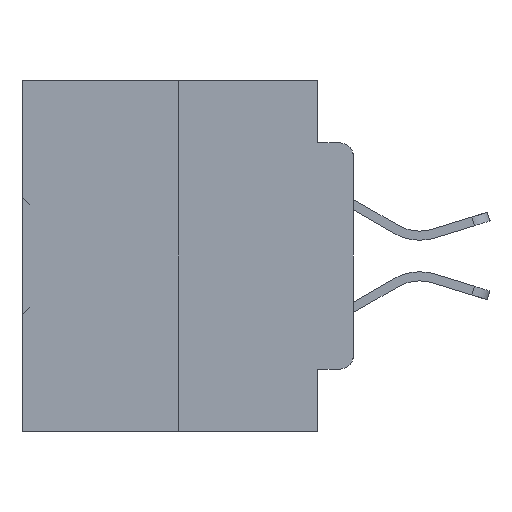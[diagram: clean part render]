
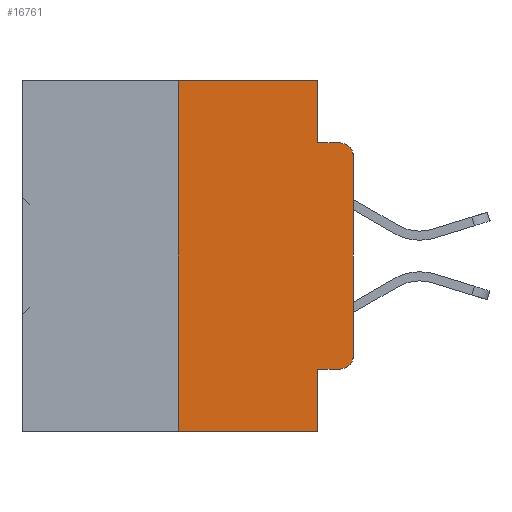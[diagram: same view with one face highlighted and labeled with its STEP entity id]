
A CAD part, left-side view. The second image highlights one B-rep face of the part: STEP entity #16761.
In plain terms, the highlighted planar face has unit normal (-1, 0, 0).
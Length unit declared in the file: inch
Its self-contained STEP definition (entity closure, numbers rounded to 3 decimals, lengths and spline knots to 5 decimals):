
#133 = CIRCLE ( 'NONE', #14691, 0.02 ) ;
#994 = CARTESIAN_POINT ( 'NONE',  ( 0., 0., -0.1085 ) ) ;
#1958 = DIRECTION ( 'NONE',  ( 0., 0., -1. ) ) ;
#3213 = AXIS2_PLACEMENT_3D ( 'NONE', #35539, #20126, #1958 ) ;
#3686 = DIRECTION ( 'NONE',  ( 0., -1., 0. ) ) ;
#3737 = ORIENTED_EDGE ( 'NONE', *, *, #10843, .F. ) ;
#4985 = ORIENTED_EDGE ( 'NONE', *, *, #38586, .T. ) ;
#5687 = EDGE_CURVE ( 'NONE', #9341, #24682, #8997, .T. ) ;
#6096 = VECTOR ( 'NONE', #7437, 39.37008 ) ;
#6361 = VERTEX_POINT ( 'NONE', #33313 ) ;
#6508 = VERTEX_POINT ( 'NONE', #19137 ) ;
#6543 = DIRECTION ( 'NONE',  ( 0., 0., -1. ) ) ;
#7009 = VECTOR ( 'NONE', #31054, 39.37008 ) ;
#7123 = ORIENTED_EDGE ( 'NONE', *, *, #9304, .F. ) ;
#7395 = DIRECTION ( 'NONE',  ( 0., 0., 1. ) ) ;
#7437 = DIRECTION ( 'NONE',  ( 0., 0., -1. ) ) ;
#7978 = FACE_OUTER_BOUND ( 'NONE', #35355, .T. ) ;
#8255 = CARTESIAN_POINT ( 'NONE',  ( 0., 0.051, -0.0885 ) ) ;
#8697 = CIRCLE ( 'NONE', #19473, 0.02 ) ;
#8997 = LINE ( 'NONE', #34598, #26923 ) ;
#9304 = EDGE_CURVE ( 'NONE', #36418, #6508, #15441, .T. ) ;
#9341 = VERTEX_POINT ( 'NONE', #22142 ) ;
#9739 = DIRECTION ( 'NONE',  ( -1., 0., 0. ) ) ;
#10552 = VECTOR ( 'NONE', #22380, 39.37008 ) ;
#10807 = EDGE_CURVE ( 'NONE', #20731, #6508, #11178, .T. ) ;
#10843 = EDGE_CURVE ( 'NONE', #20731, #35156, #24313, .T. ) ;
#11178 = LINE ( 'NONE', #24862, #33299 ) ;
#12107 = EDGE_CURVE ( 'NONE', #24682, #6361, #133, .T. ) ;
#12448 = DIRECTION ( 'NONE',  ( 0., 0., -1. ) ) ;
#13386 = CARTESIAN_POINT ( 'NONE',  ( 0., 0.02, -0.1085 ) ) ;
#13577 = CARTESIAN_POINT ( 'NONE',  ( 0., 0.051, 0. ) ) ;
#14691 = AXIS2_PLACEMENT_3D ( 'NONE', #13386, #18369, #12448 ) ;
#15061 = CARTESIAN_POINT ( 'NONE',  ( 0., 0.25, 0. ) ) ;
#15441 = LINE ( 'NONE', #29222, #6096 ) ;
#16761 = ADVANCED_FACE ( 'NONE', ( #7978 ), #19984, .F. ) ;
#17739 = CARTESIAN_POINT ( 'NONE',  ( 0., 0.02, -0.4115 ) ) ;
#18055 = ORIENTED_EDGE ( 'NONE', *, *, #31976, .F. ) ;
#18369 = DIRECTION ( 'NONE',  ( -1., 0., 0. ) ) ;
#18503 = CARTESIAN_POINT ( 'NONE',  ( 0., 0.473, 0. ) ) ;
#19137 = CARTESIAN_POINT ( 'NONE',  ( 0., 0.051, -0.5 ) ) ;
#19473 = AXIS2_PLACEMENT_3D ( 'NONE', #27525, #9739, #36559 ) ;
#19984 = PLANE ( 'NONE',  #3213 ) ;
#20126 = DIRECTION ( 'NONE',  ( 1., 0., 0. ) ) ;
#20128 = VECTOR ( 'NONE', #6543, 39.37008 ) ;
#20731 = VERTEX_POINT ( 'NONE', #25980 ) ;
#22142 = CARTESIAN_POINT ( 'NONE',  ( 0., 0., -0.3915 ) ) ;
#22200 = VECTOR ( 'NONE', #29335, 39.37008 ) ;
#22233 = CARTESIAN_POINT ( 'NONE',  ( 0., 0.051, -0.4115 ) ) ;
#22380 = DIRECTION ( 'NONE',  ( 0., -1., 0. ) ) ;
#22462 = ORIENTED_EDGE ( 'NONE', *, *, #12107, .T. ) ;
#22545 = CARTESIAN_POINT ( 'NONE',  ( 0., 0.25, 0. ) ) ;
#24021 = VERTEX_POINT ( 'NONE', #36001 ) ;
#24313 = LINE ( 'NONE', #22545, #25234 ) ;
#24682 = VERTEX_POINT ( 'NONE', #994 ) ;
#24862 = CARTESIAN_POINT ( 'NONE',  ( 0., 0.473, -0.5 ) ) ;
#25186 = EDGE_CURVE ( 'NONE', #36418, #35032, #37851, .T. ) ;
#25234 = VECTOR ( 'NONE', #7395, 39.37008 ) ;
#25931 = LINE ( 'NONE', #18503, #7009 ) ;
#25980 = CARTESIAN_POINT ( 'NONE',  ( 0., 0.25, -0.5 ) ) ;
#26680 = ORIENTED_EDGE ( 'NONE', *, *, #35970, .F. ) ;
#26923 = VECTOR ( 'NONE', #31730, 39.37008 ) ;
#27463 = CARTESIAN_POINT ( 'NONE',  ( 0., 0.051, -0.4115 ) ) ;
#27525 = CARTESIAN_POINT ( 'NONE',  ( 0., 0.02, -0.3915 ) ) ;
#28829 = EDGE_CURVE ( 'NONE', #24021, #34679, #36561, .T. ) ;
#29222 = CARTESIAN_POINT ( 'NONE',  ( 0., 0.051, 0. ) ) ;
#29335 = DIRECTION ( 'NONE',  ( 0., -1., 0. ) ) ;
#30664 = LINE ( 'NONE', #8255, #22200 ) ;
#31008 = ORIENTED_EDGE ( 'NONE', *, *, #5687, .T. ) ;
#31054 = DIRECTION ( 'NONE',  ( 0., -1., 0. ) ) ;
#31730 = DIRECTION ( 'NONE',  ( 0., 0., 1. ) ) ;
#31734 = ORIENTED_EDGE ( 'NONE', *, *, #28829, .F. ) ;
#31976 = EDGE_CURVE ( 'NONE', #34679, #6361, #30664, .T. ) ;
#33299 = VECTOR ( 'NONE', #3686, 39.37008 ) ;
#33313 = CARTESIAN_POINT ( 'NONE',  ( 0., 0.02, -0.0885 ) ) ;
#33739 = ORIENTED_EDGE ( 'NONE', *, *, #25186, .T. ) ;
#34423 = ORIENTED_EDGE ( 'NONE', *, *, #10807, .T. ) ;
#34490 = CARTESIAN_POINT ( 'NONE',  ( 0., 0.051, -0.0885 ) ) ;
#34598 = CARTESIAN_POINT ( 'NONE',  ( 0., 0., 0. ) ) ;
#34679 = VERTEX_POINT ( 'NONE', #34490 ) ;
#35032 = VERTEX_POINT ( 'NONE', #17739 ) ;
#35156 = VERTEX_POINT ( 'NONE', #15061 ) ;
#35355 = EDGE_LOOP ( 'NONE', ( #31008, #22462, #18055, #31734, #26680, #3737, #34423, #7123, #33739, #4985 ) ) ;
#35539 = CARTESIAN_POINT ( 'NONE',  ( 0., 0.473, 0. ) ) ;
#35970 = EDGE_CURVE ( 'NONE', #35156, #24021, #25931, .T. ) ;
#36001 = CARTESIAN_POINT ( 'NONE',  ( 0., 0.051, 0. ) ) ;
#36418 = VERTEX_POINT ( 'NONE', #27463 ) ;
#36559 = DIRECTION ( 'NONE',  ( 0., 0., -1. ) ) ;
#36561 = LINE ( 'NONE', #13577, #20128 ) ;
#37851 = LINE ( 'NONE', #22233, #10552 ) ;
#38586 = EDGE_CURVE ( 'NONE', #35032, #9341, #8697, .T. ) ;
